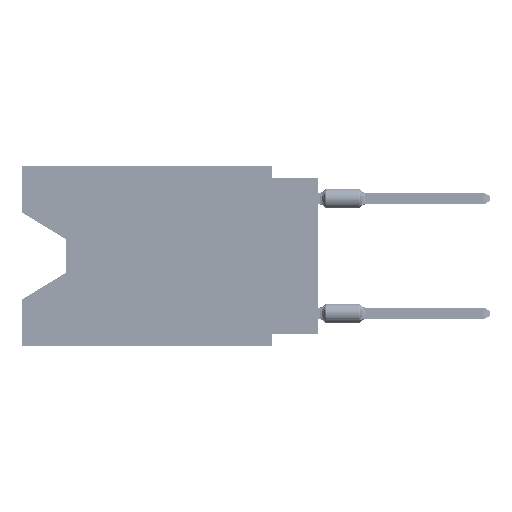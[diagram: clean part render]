
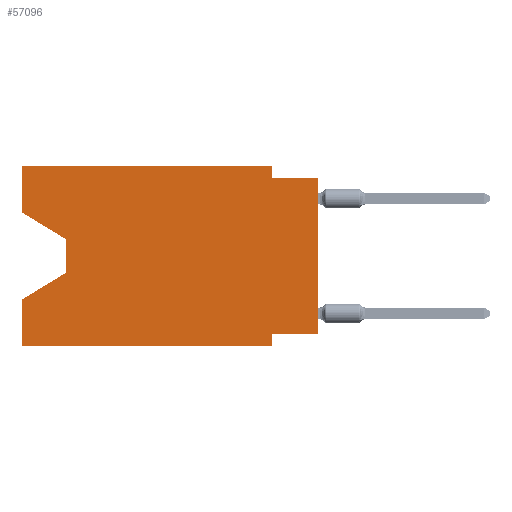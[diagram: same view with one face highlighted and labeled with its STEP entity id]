
A CAD part, left-side view. The second image highlights one B-rep face of the part: STEP entity #57096.
In plain terms, the highlighted planar face has unit normal (-1, 0, 0).
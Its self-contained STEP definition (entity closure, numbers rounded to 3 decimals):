
#1410 = VECTOR ( 'NONE', #24150, 1000. ) ;
#1940 = CARTESIAN_POINT ( 'NONE',  ( 0., 2.54, 0. ) ) ;
#1981 = EDGE_CURVE ( 'NONE', #28311, #49789, #29154, .T. ) ;
#2271 = ORIENTED_EDGE ( 'NONE', *, *, #24337, .T. ) ;
#2751 = CARTESIAN_POINT ( 'NONE',  ( 0., 2.54, -9.906 ) ) ;
#3046 = AXIS2_PLACEMENT_3D ( 'NONE', #15055, #47526, #58909 ) ;
#3321 = FACE_OUTER_BOUND ( 'NONE', #60460, .T. ) ;
#4226 = CARTESIAN_POINT ( 'NONE',  ( 0., 13.97, -4.013 ) ) ;
#4926 = ORIENTED_EDGE ( 'NONE', *, *, #60148, .F. ) ;
#6032 = ORIENTED_EDGE ( 'NONE', *, *, #45128, .F. ) ;
#6352 = CARTESIAN_POINT ( 'NONE',  ( 0., 2.54, 0. ) ) ;
#7095 = CARTESIAN_POINT ( 'NONE',  ( 0., 16.383, 0. ) ) ;
#8085 = LINE ( 'NONE', #2751, #66617 ) ;
#8580 = EDGE_CURVE ( 'NONE', #59587, #30143, #9557, .T. ) ;
#8600 = ORIENTED_EDGE ( 'NONE', *, *, #37604, .F. ) ;
#8744 = CARTESIAN_POINT ( 'NONE',  ( 0., 2.54, -9.271 ) ) ;
#8853 = EDGE_CURVE ( 'NONE', #48599, #30143, #8085, .T. ) ;
#9557 = LINE ( 'NONE', #32013, #54207 ) ;
#10070 = VERTEX_POINT ( 'NONE', #68679 ) ;
#10891 = ORIENTED_EDGE ( 'NONE', *, *, #19869, .T. ) ;
#11095 = EDGE_CURVE ( 'NONE', #58161, #42315, #62678, .T. ) ;
#13020 = LINE ( 'NONE', #45486, #53393 ) ;
#15055 = CARTESIAN_POINT ( 'NONE',  ( 0., 16.383, 0. ) ) ;
#18188 = CARTESIAN_POINT ( 'NONE',  ( 0., 0., -9.271 ) ) ;
#18693 = CARTESIAN_POINT ( 'NONE',  ( 0., 16.383, -2.546 ) ) ;
#18846 = DIRECTION ( 'NONE',  ( 0., -1., 0. ) ) ;
#18988 = VECTOR ( 'NONE', #41656, 1000. ) ;
#19869 = EDGE_CURVE ( 'NONE', #64293, #54264, #68740, .T. ) ;
#20837 = LINE ( 'NONE', #36193, #60955 ) ;
#21099 = CARTESIAN_POINT ( 'NONE',  ( 0., 0., -9.271 ) ) ;
#21153 = CARTESIAN_POINT ( 'NONE',  ( 0., 0., -0.635 ) ) ;
#21975 = VERTEX_POINT ( 'NONE', #18693 ) ;
#24150 = DIRECTION ( 'NONE',  ( 0., 0., -1. ) ) ;
#24337 = EDGE_CURVE ( 'NONE', #40524, #58161, #53073, .T. ) ;
#25624 = CARTESIAN_POINT ( 'NONE',  ( 0., 13.97, -5.893 ) ) ;
#27266 = VECTOR ( 'NONE', #42029, 1000. ) ;
#28311 = VERTEX_POINT ( 'NONE', #1940 ) ;
#28641 = CARTESIAN_POINT ( 'NONE',  ( 0., 16.383, 0. ) ) ;
#29092 = VECTOR ( 'NONE', #35965, 1000. ) ;
#29154 = LINE ( 'NONE', #6352, #1410 ) ;
#30143 = VERTEX_POINT ( 'NONE', #40272 ) ;
#31669 = DIRECTION ( 'NONE',  ( 0., -1., 0. ) ) ;
#32013 = CARTESIAN_POINT ( 'NONE',  ( 0., 16.383, -9.906 ) ) ;
#32158 = DIRECTION ( 'NONE',  ( 0., 1., 0. ) ) ;
#32358 = ORIENTED_EDGE ( 'NONE', *, *, #8580, .T. ) ;
#33633 = DIRECTION ( 'NONE',  ( 0., -1., 0. ) ) ;
#34704 = LINE ( 'NONE', #28641, #70271 ) ;
#35564 = VECTOR ( 'NONE', #18846, 1000. ) ;
#35965 = DIRECTION ( 'NONE',  ( 0., 0., 1. ) ) ;
#36193 = CARTESIAN_POINT ( 'NONE',  ( 0., 16.383, -2.546 ) ) ;
#36375 = CARTESIAN_POINT ( 'NONE',  ( 0., 13.97, -4.013 ) ) ;
#37407 = ORIENTED_EDGE ( 'NONE', *, *, #60844, .F. ) ;
#37564 = LINE ( 'NONE', #21153, #49131 ) ;
#37604 = EDGE_CURVE ( 'NONE', #49789, #54264, #37564, .T. ) ;
#40272 = CARTESIAN_POINT ( 'NONE',  ( 0., 2.54, -9.906 ) ) ;
#40524 = VERTEX_POINT ( 'NONE', #36375 ) ;
#40740 = EDGE_CURVE ( 'NONE', #10070, #28311, #51300, .T. ) ;
#40817 = ORIENTED_EDGE ( 'NONE', *, *, #8853, .F. ) ;
#41340 = ORIENTED_EDGE ( 'NONE', *, *, #1981, .F. ) ;
#41656 = DIRECTION ( 'NONE',  ( 0., 0.855, -0.519 ) ) ;
#42029 = DIRECTION ( 'NONE',  ( 0., 0., -1. ) ) ;
#42315 = VERTEX_POINT ( 'NONE', #57804 ) ;
#42859 = CARTESIAN_POINT ( 'NONE',  ( 0., 16.383, -9.906 ) ) ;
#44305 = ORIENTED_EDGE ( 'NONE', *, *, #11095, .T. ) ;
#45128 = EDGE_CURVE ( 'NONE', #21975, #10070, #34704, .T. ) ;
#45486 = CARTESIAN_POINT ( 'NONE',  ( 0., 16.383, 0. ) ) ;
#46670 = CARTESIAN_POINT ( 'NONE',  ( 0., 0., 0. ) ) ;
#46827 = PLANE ( 'NONE',  #3046 ) ;
#47526 = DIRECTION ( 'NONE',  ( 1., 0., 0. ) ) ;
#47771 = VECTOR ( 'NONE', #32158, 1000. ) ;
#48599 = VERTEX_POINT ( 'NONE', #8744 ) ;
#49131 = VECTOR ( 'NONE', #33633, 1000. ) ;
#49160 = ORIENTED_EDGE ( 'NONE', *, *, #70333, .T. ) ;
#49789 = VERTEX_POINT ( 'NONE', #59160 ) ;
#51300 = LINE ( 'NONE', #7095, #35564 ) ;
#53073 = LINE ( 'NONE', #4226, #27266 ) ;
#53287 = DIRECTION ( 'NONE',  ( 0., -0.855, -0.519 ) ) ;
#53393 = VECTOR ( 'NONE', #56170, 1000. ) ;
#54207 = VECTOR ( 'NONE', #31669, 1000. ) ;
#54264 = VERTEX_POINT ( 'NONE', #57498 ) ;
#54958 = LINE ( 'NONE', #21099, #47771 ) ;
#55737 = DIRECTION ( 'NONE',  ( 0., 0., 1. ) ) ;
#56170 = DIRECTION ( 'NONE',  ( 0., 0., 1. ) ) ;
#56928 = DIRECTION ( 'NONE',  ( 0., 0., -1. ) ) ;
#57096 = ADVANCED_FACE ( 'NONE', ( #3321 ), #46827, .F. ) ;
#57498 = CARTESIAN_POINT ( 'NONE',  ( 0., 0., -0.635 ) ) ;
#57804 = CARTESIAN_POINT ( 'NONE',  ( 0., 16.383, -7.36 ) ) ;
#58161 = VERTEX_POINT ( 'NONE', #25624 ) ;
#58909 = DIRECTION ( 'NONE',  ( 0., 0., -1. ) ) ;
#59160 = CARTESIAN_POINT ( 'NONE',  ( 0., 2.54, -0.635 ) ) ;
#59587 = VERTEX_POINT ( 'NONE', #42859 ) ;
#60148 = EDGE_CURVE ( 'NONE', #59587, #42315, #13020, .T. ) ;
#60460 = EDGE_LOOP ( 'NONE', ( #49160, #2271, #44305, #4926, #32358, #40817, #37407, #10891, #8600, #41340, #67677, #6032 ) ) ;
#60844 = EDGE_CURVE ( 'NONE', #64293, #48599, #54958, .T. ) ;
#60955 = VECTOR ( 'NONE', #53287, 1000. ) ;
#61969 = CARTESIAN_POINT ( 'NONE',  ( 0., 13.97, -5.893 ) ) ;
#62678 = LINE ( 'NONE', #61969, #18988 ) ;
#64293 = VERTEX_POINT ( 'NONE', #18188 ) ;
#66617 = VECTOR ( 'NONE', #56928, 1000. ) ;
#67677 = ORIENTED_EDGE ( 'NONE', *, *, #40740, .F. ) ;
#68679 = CARTESIAN_POINT ( 'NONE',  ( 0., 16.383, 0. ) ) ;
#68740 = LINE ( 'NONE', #46670, #29092 ) ;
#70271 = VECTOR ( 'NONE', #55737, 1000. ) ;
#70333 = EDGE_CURVE ( 'NONE', #21975, #40524, #20837, .T. ) ;
